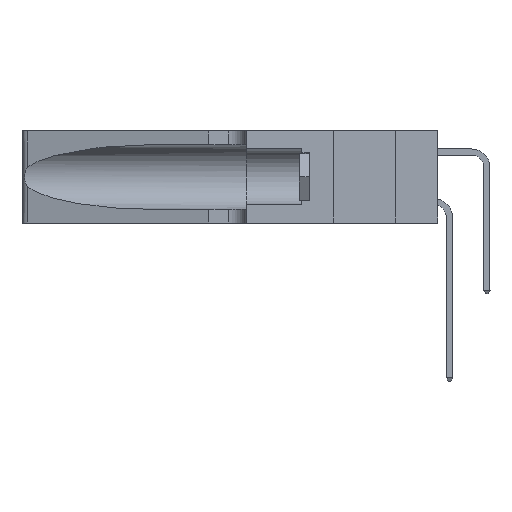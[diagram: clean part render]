
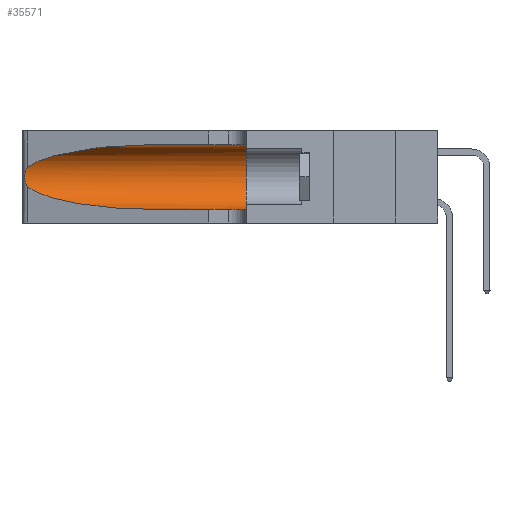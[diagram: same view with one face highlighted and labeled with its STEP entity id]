
A CAD part, left-side view. The second image highlights one B-rep face of the part: STEP entity #35571.
In plain terms, the highlighted cylindrical face has radius 3.308 mm (diameter 6.617 mm), a partial arc.
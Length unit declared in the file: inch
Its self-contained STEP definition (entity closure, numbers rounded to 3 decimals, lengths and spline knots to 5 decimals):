
#730 = EDGE_CURVE ( 'NONE', #16632, #28699, #26330, .T. ) ;
#1687 = FACE_OUTER_BOUND ( 'NONE', #13349, .T. ) ;
#1750 = CARTESIAN_POINT ( 'NONE',  ( 0.1305, 1.61858, 0.05475 ) ) ;
#2099 = EDGE_CURVE ( 'NONE', #6171, #17362, #33150, .T. ) ;
#2622 = CYLINDRICAL_SURFACE ( 'NONE', #26216, 0.13025 ) ;
#2831 = CARTESIAN_POINT ( 'NONE',  ( 0.1305, 0.72297, 0.05475 ) ) ;
#3058 = EDGE_CURVE ( 'NONE', #5764, #24877, #21496, .T. ) ;
#3498 = LINE ( 'NONE', #1750, #31470 ) ;
#4731 = CARTESIAN_POINT ( 'NONE',  ( 0.25487, 1.22718, 0.14631 ) ) ;
#5764 = VERTEX_POINT ( 'NONE', #25184 ) ;
#6028 = EDGE_CURVE ( 'NONE', #28699, #6171, #30535, .T. ) ;
#6171 = VERTEX_POINT ( 'NONE', #10240 ) ;
#6675 = EDGE_CURVE ( 'NONE', #17362, #24877, #3498, .T. ) ;
#6910 = CARTESIAN_POINT ( 'NONE',  ( 0.1305, 0.72297, 0.31525 ) ) ;
#7173 = CARTESIAN_POINT ( 'NONE',  ( 0.1305, 0.72297, 0.31525 ) ) ;
#8382 = DIRECTION ( 'NONE',  ( 0., 1., 0. ) ) ;
#8496 = ORIENTED_EDGE ( 'NONE', *, *, #2099, .T. ) ;
#9598 = CARTESIAN_POINT ( 'NONE',  ( 0.25854, 1.2359, 0.20912 ) ) ;
#10210 = CARTESIAN_POINT ( 'NONE',  ( 0.25856, 1.23593, 0.16098 ) ) ;
#10240 = CARTESIAN_POINT ( 'NONE',  ( 0.25487, 1.22718, 0.14631 ) ) ;
#10268 = CARTESIAN_POINT ( 'NONE',  ( 0.2373, 1.15595, 0.08982 ) ) ;
#10750 = CARTESIAN_POINT ( 'NONE',  ( 0.1305, 0.72297, 0.05475 ) ) ;
#10873 = CARTESIAN_POINT ( 'NONE',  ( 0.1305, 0.35, 0.185 ) ) ;
#11653 = VECTOR ( 'NONE', #34964, 39.37008 ) ;
#12340 = CARTESIAN_POINT ( 'NONE',  ( 0.26075, 1.23896, 0.19203 ) ) ;
#12510 = ORIENTED_EDGE ( 'NONE', *, *, #730, .T. ) ;
#12581 = DIRECTION ( 'NONE',  ( 0., -1., 0. ) ) ;
#12992 = CARTESIAN_POINT ( 'NONE',  ( 0.25789, 1.23486, 0.15765 ) ) ;
#13349 = EDGE_LOOP ( 'NONE', ( #12510, #22422, #8496, #18577, #32173, #28396 ) ) ;
#15381 = CARTESIAN_POINT ( 'NONE',  ( 0.25555, 1.22993, 0.14849 ) ) ;
#16559 = CARTESIAN_POINT ( 'NONE',  ( 0.1305, 0.35, 0.05475 ) ) ;
#16632 = VERTEX_POINT ( 'NONE', #6910 ) ;
#17362 = VERTEX_POINT ( 'NONE', #2831 ) ;
#18577 = ORIENTED_EDGE ( 'NONE', *, *, #6675, .T. ) ;
#18920 = CARTESIAN_POINT ( 'NONE',  ( 0.18966, 0.96281, 0.05475 ) ) ;
#20332 = EDGE_CURVE ( 'NONE', #16632, #5764, #28037, .T. ) ;
#20917 = CARTESIAN_POINT ( 'NONE',  ( 0.25639, 1.23186, 0.15144 ) ) ;
#21258 = CARTESIAN_POINT ( 'NONE',  ( 0.26017, 1.23833, 0.17102 ) ) ;
#21496 = CIRCLE ( 'NONE', #31333, 0.13025 ) ;
#22422 = ORIENTED_EDGE ( 'NONE', *, *, #6028, .T. ) ;
#23130 = DIRECTION ( 'NONE',  ( 0., 0., -1. ) ) ;
#23318 = CARTESIAN_POINT ( 'NONE',  ( 0.25639, 1.23184, 0.21858 ) ) ;
#23453 = CARTESIAN_POINT ( 'NONE',  ( 0.25555, 1.22994, 0.2215 ) ) ;
#23705 = CARTESIAN_POINT ( 'NONE',  ( 0.1305, 1.61858, 0.31525 ) ) ;
#23710 = CARTESIAN_POINT ( 'NONE',  ( 0.25487, 1.22718, 0.22369 ) ) ;
#24267 = CARTESIAN_POINT ( 'NONE',  ( 0.25487, 1.22718, 0.22369 ) ) ;
#24877 = VERTEX_POINT ( 'NONE', #16559 ) ;
#25184 = CARTESIAN_POINT ( 'NONE',  ( 0.1305, 0.35, 0.31525 ) ) ;
#26083 = CARTESIAN_POINT ( 'NONE',  ( 0.25787, 1.23484, 0.2124 ) ) ;
#26216 = AXIS2_PLACEMENT_3D ( 'NONE', #31802, #28913, #23130 ) ;
#26330 =( BOUNDED_CURVE ( )  B_SPLINE_CURVE ( 3, ( #7173, #26407, #31920, #34906 ),
 .UNSPECIFIED., .F., .T. ) 
 B_SPLINE_CURVE_WITH_KNOTS ( ( 4, 4 ),
 ( 1.5708, 2.84003 ),
 .UNSPECIFIED. ) 
 CURVE ( )  GEOMETRIC_REPRESENTATION_ITEM ( )  RATIONAL_B_SPLINE_CURVE ( ( 1., 0.87, 0.87, 1. ) ) 
 REPRESENTATION_ITEM ( '' )  );
#26407 = CARTESIAN_POINT ( 'NONE',  ( 0.18966, 0.96281, 0.31525 ) ) ;
#27593 = DIRECTION ( 'NONE',  ( 0., 0., 1. ) ) ;
#28037 = LINE ( 'NONE', #23705, #11653 ) ;
#28396 = ORIENTED_EDGE ( 'NONE', *, *, #20332, .F. ) ;
#28699 = VERTEX_POINT ( 'NONE', #24267 ) ;
#28834 = CARTESIAN_POINT ( 'NONE',  ( 0.26018, 1.23835, 0.19895 ) ) ;
#28913 = DIRECTION ( 'NONE',  ( 0., -1., 0. ) ) ;
#30535 = B_SPLINE_CURVE_WITH_KNOTS ( 'NONE', 3,
 ( #23710, #23453, #23318, #26083, #9598, #28834, #12340, #34342, #21258, #10210, #12992, #20917, #15381, #32211 ),
 .UNSPECIFIED., .F., .F.,
 ( 4, 2, 2, 2, 2, 2, 4 ),
 ( 0., 0.00027, 0.00053, 0.00107, 0.0016, 0.00187, 0.00214 ),
 .UNSPECIFIED. ) ;
#31333 = AXIS2_PLACEMENT_3D ( 'NONE', #10873, #8382, #27593 ) ;
#31470 = VECTOR ( 'NONE', #12581, 39.37008 ) ;
#31802 = CARTESIAN_POINT ( 'NONE',  ( 0.1305, 1.61858, 0.185 ) ) ;
#31920 = CARTESIAN_POINT ( 'NONE',  ( 0.2373, 1.15595, 0.28018 ) ) ;
#32173 = ORIENTED_EDGE ( 'NONE', *, *, #3058, .F. ) ;
#32211 = CARTESIAN_POINT ( 'NONE',  ( 0.25487, 1.22718, 0.14631 ) ) ;
#33150 =( BOUNDED_CURVE ( )  B_SPLINE_CURVE ( 3, ( #4731, #10268, #18920, #10750 ),
 .UNSPECIFIED., .F., .T. ) 
 B_SPLINE_CURVE_WITH_KNOTS ( ( 4, 4 ),
 ( 3.44316, 4.71239 ),
 .UNSPECIFIED. ) 
 CURVE ( )  GEOMETRIC_REPRESENTATION_ITEM ( )  RATIONAL_B_SPLINE_CURVE ( ( 1., 0.87, 0.87, 1. ) ) 
 REPRESENTATION_ITEM ( '' )  );
#34342 = CARTESIAN_POINT ( 'NONE',  ( 0.26075, 1.23896, 0.178 ) ) ;
#34906 = CARTESIAN_POINT ( 'NONE',  ( 0.25487, 1.22718, 0.22369 ) ) ;
#34964 = DIRECTION ( 'NONE',  ( 0., -1., 0. ) ) ;
#35571 = ADVANCED_FACE ( 'NONE', ( #1687 ), #2622, .F. ) ;
